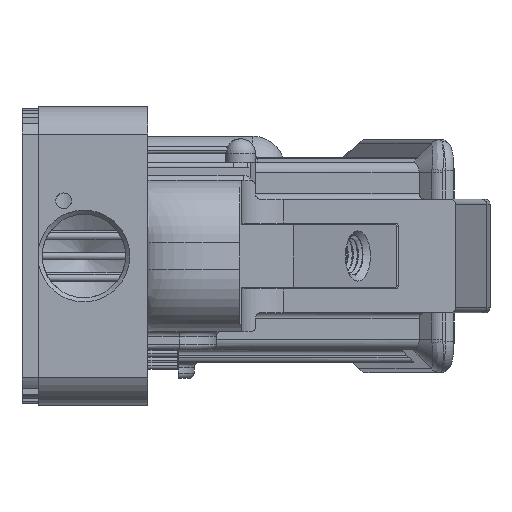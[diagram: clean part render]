
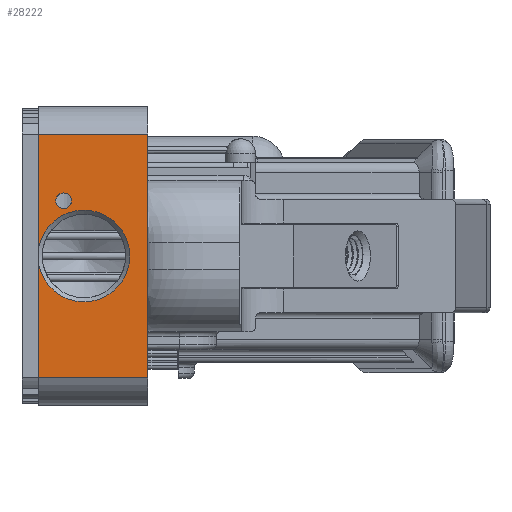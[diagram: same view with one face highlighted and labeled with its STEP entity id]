
A CAD part, left-side view. The second image highlights one B-rep face of the part: STEP entity #28222.
In plain terms, the highlighted planar face has unit normal (-1, 0, 0).
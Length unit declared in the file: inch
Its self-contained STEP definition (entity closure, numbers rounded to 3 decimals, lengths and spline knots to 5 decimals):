
#2215=VECTOR('',#30526,1.);
#2216=VECTOR('',#30527,1.);
#2563=VECTOR('',#31951,1.);
#2565=VECTOR('',#31954,1.);
#2740=VECTOR('',#32477,1.);
#2848=VECTOR('',#32711,1.);
#2851=VECTOR('',#32720,1.);
#2867=VECTOR('',#32842,1.);
#2868=VECTOR('',#32843,1.);
#3782=LINE('',#36468,#2215);
#3783=LINE('',#36474,#2216);
#4130=LINE('',#50500,#2563);
#4132=LINE('',#50505,#2565);
#4307=LINE('',#52899,#2740);
#4415=LINE('',#54062,#2848);
#4418=LINE('',#54072,#2851);
#4434=LINE('',#70209,#2867);
#4435=LINE('',#70210,#2868);
#5302=PLANE('',#79249);
#6006=VERTEX_POINT('',#36467);
#6007=VERTEX_POINT('',#36469);
#6008=VERTEX_POINT('',#36473);
#6009=VERTEX_POINT('',#36475);
#7057=VERTEX_POINT('',#50491);
#7059=VERTEX_POINT('',#50495);
#7061=VERTEX_POINT('',#50499);
#7062=VERTEX_POINT('',#50503);
#7064=VERTEX_POINT('',#50506);
#7316=VERTEX_POINT('',#52900);
#7522=VERTEX_POINT('',#54071);
#8967=CIRCLE('',#78899,0.047);
#9121=CIRCLE('',#79248,0.275);
#10171=EDGE_CURVE('',#6007,#6006,#3782,.T.);
#10173=EDGE_CURVE('',#6009,#6008,#3783,.T.);
#11509=EDGE_CURVE('',#7057,#7057,#8967,.T.);
#11513=EDGE_CURVE('',#7059,#7061,#4130,.T.);
#11515=EDGE_CURVE('',#7062,#7064,#4132,.T.);
#11854=EDGE_CURVE('',#7316,#7064,#4307,.T.);
#12087=EDGE_CURVE('',#7062,#7059,#4415,.F.);
#12092=EDGE_CURVE('',#7061,#7522,#4418,.T.);
#12306=EDGE_CURVE('',#6007,#6008,#9121,.T.);
#12307=EDGE_CURVE('',#6006,#7316,#4434,.T.);
#12308=EDGE_CURVE('',#7522,#6009,#4435,.T.);
#18346=ORIENTED_EDGE('',*,*,#10171,.T.);
#18347=ORIENTED_EDGE('',*,*,#12307,.T.);
#18348=ORIENTED_EDGE('',*,*,#11854,.T.);
#18349=ORIENTED_EDGE('',*,*,#11515,.F.);
#18350=ORIENTED_EDGE('',*,*,#12087,.T.);
#18351=ORIENTED_EDGE('',*,*,#11513,.T.);
#18352=ORIENTED_EDGE('',*,*,#12092,.T.);
#18353=ORIENTED_EDGE('',*,*,#12308,.T.);
#18354=ORIENTED_EDGE('',*,*,#10173,.T.);
#18355=ORIENTED_EDGE('',*,*,#12306,.F.);
#18356=ORIENTED_EDGE('',*,*,#11509,.T.);
#23220=EDGE_LOOP('',(#18346,#18347,#18348,#18349,#18350,#18351,#18352,#18353,
#18354,#18355));
#23221=EDGE_LOOP('',(#18356));
#25907=FACE_BOUND('',#23220,.T.);
#25908=FACE_BOUND('',#23221,.T.);
#28222=ADVANCED_FACE('',(#25907,#25908),#5302,.F.);
#30526=DIRECTION('',(0.,0.,-1.));
#30527=DIRECTION('',(0.,0.,-1.));
#31945=DIRECTION('',(1.,0.,0.));
#31946=DIRECTION('',(0.,0.,0.047));
#31951=DIRECTION('',(0.,-1.,0.));
#31954=DIRECTION('',(0.,-1.,0.));
#32477=DIRECTION('',(0.,0.,1.));
#32711=DIRECTION('',(0.,0.,-1.));
#32720=DIRECTION('',(0.,0.,1.));
#32839=DIRECTION('',(-1.,0.,0.));
#32840=DIRECTION('',(0.,0.,-0.275));
#32841=DIRECTION('',(1.,0.,0.));
#32842=DIRECTION('',(0.,-1.,0.));
#32843=DIRECTION('',(0.,1.,0.));
#36467=CARTESIAN_POINT('',(-7.503,0.1505,-0.73097));
#36468=CARTESIAN_POINT('',(-7.503,0.1505,0.02765));
#36469=CARTESIAN_POINT('',(-7.503,0.1505,-0.04673));
#36473=CARTESIAN_POINT('',(-7.503,0.1505,0.04673));
#36474=CARTESIAN_POINT('',(-7.503,0.1505,0.02765));
#36475=CARTESIAN_POINT('',(-7.503,0.1505,0.73097));
#50490=CARTESIAN_POINT('',(-7.503,0.0005,0.331));
#50491=CARTESIAN_POINT('',(-7.503,0.0005,0.378));
#50495=CARTESIAN_POINT('',(-7.503,-0.5045,0.37638));
#50499=CARTESIAN_POINT('',(-7.503,-0.50466,0.37638));
#50500=CARTESIAN_POINT('',(-7.503,-0.22666,0.37638));
#50503=CARTESIAN_POINT('',(-7.503,-0.5045,-0.37638));
#50505=CARTESIAN_POINT('',(-7.503,-0.22666,-0.37638));
#50506=CARTESIAN_POINT('',(-7.503,-0.50466,-0.37638));
#52899=CARTESIAN_POINT('',(-7.503,-0.50466,-0.73097));
#52900=CARTESIAN_POINT('',(-7.503,-0.50466,-0.73097));
#54062=CARTESIAN_POINT('',(-7.503,-0.5045,-0.22588));
#54071=CARTESIAN_POINT('',(-7.503,-0.50466,0.73097));
#54072=CARTESIAN_POINT('',(-7.503,-0.50466,0.73097));
#70207=CARTESIAN_POINT('',(-7.503,-0.1205,0.));
#70208=CARTESIAN_POINT('',(-7.503,-0.55779,0.00136));
#70209=CARTESIAN_POINT('',(-7.503,-0.39222,-0.73097));
#70210=CARTESIAN_POINT('',(-7.503,0.1505,0.73097));
#78899=AXIS2_PLACEMENT_3D('',#50490,#31945,#31946);
#79248=AXIS2_PLACEMENT_3D('',#70207,#32839,#32840);
#79249=AXIS2_PLACEMENT_3D('',#70208,#32841,$);
